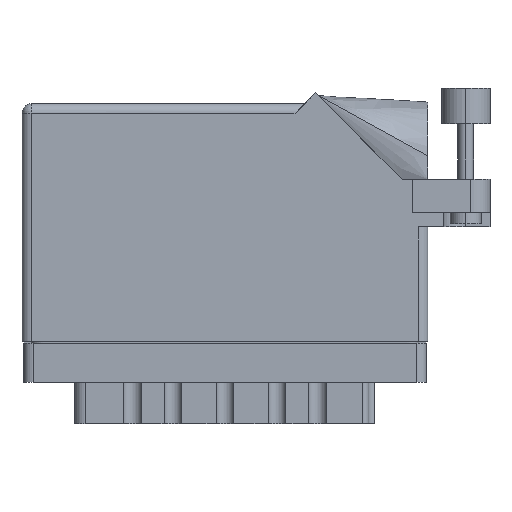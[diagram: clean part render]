
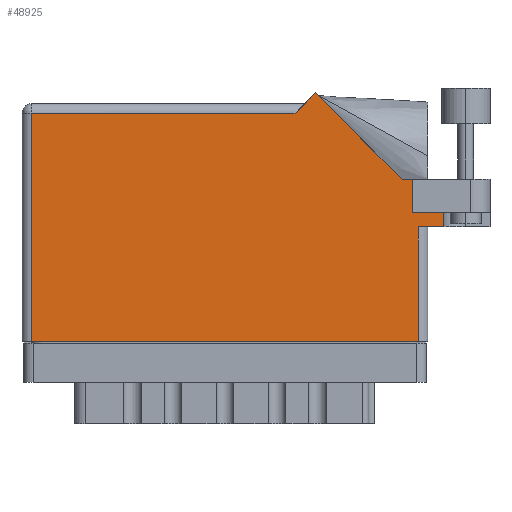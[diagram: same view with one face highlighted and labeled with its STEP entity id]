
A CAD part, front view. The second image highlights one B-rep face of the part: STEP entity #48925.
In plain terms, the highlighted face is planar.
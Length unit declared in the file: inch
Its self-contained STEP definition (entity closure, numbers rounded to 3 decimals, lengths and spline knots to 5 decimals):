
#1061 = CARTESIAN_POINT ( 'NONE',  ( 2.7135, 0.737, 0. ) ) ;
#1137 = EDGE_CURVE ( 'NONE', #4296, #29913, #32635, .T. ) ;
#1673 = ORIENTED_EDGE ( 'NONE', *, *, #6007, .T. ) ;
#3181 = CARTESIAN_POINT ( 'NONE',  ( 2.44642, 1.044, 0. ) ) ;
#3701 = LINE ( 'NONE', #31021, #6699 ) ;
#4086 = LINE ( 'NONE', #41255, #40523 ) ;
#4296 = VERTEX_POINT ( 'NONE', #45730 ) ;
#5792 = DIRECTION ( 'NONE',  ( 0., -1., 0. ) ) ;
#6007 = EDGE_CURVE ( 'NONE', #36122, #37868, #13078, .T. ) ;
#6261 = VECTOR ( 'NONE', #16459, 39.37008 ) ;
#6585 = VERTEX_POINT ( 'NONE', #11233 ) ;
#6699 = VECTOR ( 'NONE', #30865, 39.37008 ) ;
#7340 = VECTOR ( 'NONE', #32224, 39.37008 ) ;
#7363 = CARTESIAN_POINT ( 'NONE',  ( 2.512, 0.831, 0. ) ) ;
#8472 = VERTEX_POINT ( 'NONE', #1061 ) ;
#8762 = EDGE_CURVE ( 'NONE', #37868, #25584, #3701, .T. ) ;
#9652 = VERTEX_POINT ( 'NONE', #3181 ) ;
#9834 = LINE ( 'NONE', #18561, #27222 ) ;
#10187 = VECTOR ( 'NONE', #45618, 39.37008 ) ;
#10234 = DIRECTION ( 'NONE',  ( -1., 0., 0. ) ) ;
#10320 = EDGE_CURVE ( 'NONE', #20876, #8472, #27428, .T. ) ;
#10490 = DIRECTION ( 'NONE',  ( 0., 0., -1. ) ) ;
#10663 = VECTOR ( 'NONE', #5792, 39.37008 ) ;
#10978 = CARTESIAN_POINT ( 'NONE',  ( 2.55, 0.737, 0. ) ) ;
#11233 = CARTESIAN_POINT ( 'NONE',  ( 2.512, 1.044, 0. ) ) ;
#12290 = VECTOR ( 'NONE', #36983, 39.37008 ) ;
#12946 = EDGE_CURVE ( 'NONE', #29913, #36122, #4086, .T. ) ;
#13078 = LINE ( 'NONE', #42856, #10663 ) ;
#13441 = EDGE_CURVE ( 'NONE', #29442, #8472, #40172, .T. ) ;
#13649 = LINE ( 'NONE', #16883, #47655 ) ;
#14979 = AXIS2_PLACEMENT_3D ( 'NONE', #37375, #10490, #41027 ) ;
#14981 = ORIENTED_EDGE ( 'NONE', *, *, #8762, .T. ) ;
#15510 = EDGE_CURVE ( 'NONE', #25584, #29442, #13649, .T. ) ;
#15961 = CARTESIAN_POINT ( 'NONE',  ( 3.012, 1.044, 0. ) ) ;
#16459 = DIRECTION ( 'NONE',  ( -1., 0., 0. ) ) ;
#16883 = CARTESIAN_POINT ( 'NONE',  ( 2.55, 0.737, 0. ) ) ;
#16916 = CARTESIAN_POINT ( 'NONE',  ( 1.757, 1.468, 0. ) ) ;
#17271 = VECTOR ( 'NONE', #39291, 39.37008 ) ;
#18055 = EDGE_CURVE ( 'NONE', #49329, #6585, #9834, .T. ) ;
#18561 = CARTESIAN_POINT ( 'NONE',  ( 2.512, 0.831, 0. ) ) ;
#19661 = ORIENTED_EDGE ( 'NONE', *, *, #12946, .T. ) ;
#19829 = FACE_OUTER_BOUND ( 'NONE', #21260, .T. ) ;
#20876 = VERTEX_POINT ( 'NONE', #27762 ) ;
#21232 = EDGE_CURVE ( 'NONE', #49329, #20876, #24069, .T. ) ;
#21260 = EDGE_LOOP ( 'NONE', ( #14981, #47773, #27890, #35202, #41571, #22162, #22348, #24511, #26460, #19661, #1673 ) ) ;
#22018 = CARTESIAN_POINT ( 'NONE',  ( 2.55, 0., 0. ) ) ;
#22020 = PLANE ( 'NONE',  #14979 ) ;
#22162 = ORIENTED_EDGE ( 'NONE', *, *, #18055, .T. ) ;
#22348 = ORIENTED_EDGE ( 'NONE', *, *, #44114, .T. ) ;
#24069 = LINE ( 'NONE', #7363, #35435 ) ;
#24511 = ORIENTED_EDGE ( 'NONE', *, *, #33877, .T. ) ;
#24957 = CARTESIAN_POINT ( 'NONE',  ( 1.819, 1.53, 0. ) ) ;
#25584 = VERTEX_POINT ( 'NONE', #22018 ) ;
#26460 = ORIENTED_EDGE ( 'NONE', *, *, #1137, .T. ) ;
#26567 = DIRECTION ( 'NONE',  ( 1., 0., 0. ) ) ;
#27222 = VECTOR ( 'NONE', #30272, 39.37008 ) ;
#27428 = LINE ( 'NONE', #39613, #17271 ) ;
#27762 = CARTESIAN_POINT ( 'NONE',  ( 2.7135, 0.831, 0. ) ) ;
#27890 = ORIENTED_EDGE ( 'NONE', *, *, #13441, .T. ) ;
#29442 = VERTEX_POINT ( 'NONE', #10978 ) ;
#29765 = CARTESIAN_POINT ( 'NONE',  ( 0.062, 0., 0. ) ) ;
#29913 = VERTEX_POINT ( 'NONE', #16916 ) ;
#30272 = DIRECTION ( 'NONE',  ( 0., 1., 0. ) ) ;
#30494 = CARTESIAN_POINT ( 'NONE',  ( 2.44642, 1.044, 0. ) ) ;
#30865 = DIRECTION ( 'NONE',  ( 1., 0., 0. ) ) ;
#31021 = CARTESIAN_POINT ( 'NONE',  ( 0., 0., 0. ) ) ;
#31907 = CARTESIAN_POINT ( 'NONE',  ( 2.612, 0.737, 0. ) ) ;
#32224 = DIRECTION ( 'NONE',  ( 1., 0., 0. ) ) ;
#32635 = LINE ( 'NONE', #24957, #12290 ) ;
#33877 = EDGE_CURVE ( 'NONE', #9652, #4296, #41210, .T. ) ;
#35202 = ORIENTED_EDGE ( 'NONE', *, *, #10320, .F. ) ;
#35435 = VECTOR ( 'NONE', #26567, 39.37008 ) ;
#36122 = VERTEX_POINT ( 'NONE', #38252 ) ;
#36157 = LINE ( 'NONE', #15961, #6261 ) ;
#36983 = DIRECTION ( 'NONE',  ( -0.707, -0.707, 0. ) ) ;
#37375 = CARTESIAN_POINT ( 'NONE',  ( 0., 1.53, 0. ) ) ;
#37868 = VERTEX_POINT ( 'NONE', #29765 ) ;
#38252 = CARTESIAN_POINT ( 'NONE',  ( 0.062, 1.468, 0. ) ) ;
#39291 = DIRECTION ( 'NONE',  ( 0., -1., 0. ) ) ;
#39613 = CARTESIAN_POINT ( 'NONE',  ( 2.7135, 1.16177, 0. ) ) ;
#40172 = LINE ( 'NONE', #31907, #7340 ) ;
#40523 = VECTOR ( 'NONE', #10234, 39.37008 ) ;
#41027 = DIRECTION ( 'NONE',  ( -1., 0., 0. ) ) ;
#41210 = LINE ( 'NONE', #30494, #10187 ) ;
#41255 = CARTESIAN_POINT ( 'NONE',  ( 0., 1.468, 0. ) ) ;
#41571 = ORIENTED_EDGE ( 'NONE', *, *, #21232, .F. ) ;
#42856 = CARTESIAN_POINT ( 'NONE',  ( 0.062, 0., 0. ) ) ;
#43585 = CARTESIAN_POINT ( 'NONE',  ( 2.512, 0.831, 0. ) ) ;
#44114 = EDGE_CURVE ( 'NONE', #6585, #9652, #36157, .T. ) ;
#45618 = DIRECTION ( 'NONE',  ( -0.707, 0.707, 0. ) ) ;
#45730 = CARTESIAN_POINT ( 'NONE',  ( 1.88971, 1.60071, 0. ) ) ;
#47405 = DIRECTION ( 'NONE',  ( 0., 1., 0. ) ) ;
#47655 = VECTOR ( 'NONE', #47405, 39.37008 ) ;
#47773 = ORIENTED_EDGE ( 'NONE', *, *, #15510, .T. ) ;
#48925 = ADVANCED_FACE ( 'NONE', ( #19829 ), #22020, .F. ) ;
#49329 = VERTEX_POINT ( 'NONE', #43585 ) ;
